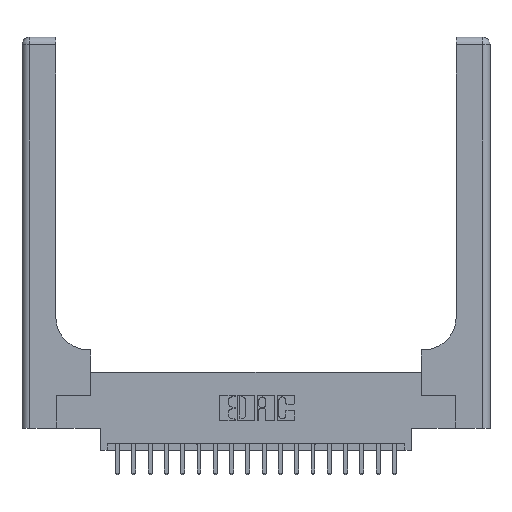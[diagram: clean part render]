
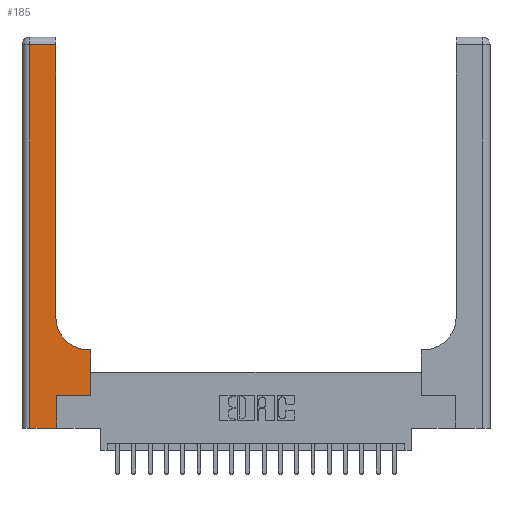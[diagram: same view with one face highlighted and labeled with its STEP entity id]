
A CAD part, top view. The second image highlights one B-rep face of the part: STEP entity #185.
In plain terms, the highlighted planar face has unit normal (0, 0, 1).
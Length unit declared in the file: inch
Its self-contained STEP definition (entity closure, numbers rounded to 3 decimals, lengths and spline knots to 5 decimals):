
#185 = ADVANCED_FACE ( 'NONE', ( #531 ), #16357, .F. ) ;
#223 = EDGE_CURVE ( 'NONE', #10310, #5953, #11863, .T. ) ;
#393 = ORIENTED_EDGE ( 'NONE', *, *, #2539, .T. ) ;
#531 = FACE_OUTER_BOUND ( 'NONE', #19480, .T. ) ;
#795 = ORIENTED_EDGE ( 'NONE', *, *, #9031, .T. ) ;
#1350 = DIRECTION ( 'NONE',  ( 0., 1., 0. ) ) ;
#1409 = ORIENTED_EDGE ( 'NONE', *, *, #223, .T. ) ;
#1670 = CARTESIAN_POINT ( 'NONE',  ( 0., 2.94, 0.37 ) ) ;
#2201 = CARTESIAN_POINT ( 'NONE',  ( 0.528, 0.25, 0.37 ) ) ;
#2447 = ORIENTED_EDGE ( 'NONE', *, *, #11754, .T. ) ;
#2539 = EDGE_CURVE ( 'NONE', #5953, #5606, #13734, .T. ) ;
#2659 = VECTOR ( 'NONE', #10276, 39.37008 ) ;
#2697 = VERTEX_POINT ( 'NONE', #13603 ) ;
#2751 = CARTESIAN_POINT ( 'NONE',  ( 0., 0., 0.37 ) ) ;
#4132 = VERTEX_POINT ( 'NONE', #9927 ) ;
#4357 = DIRECTION ( 'NONE',  ( 1., 0., 0. ) ) ;
#4760 = VECTOR ( 'NONE', #1350, 39.37008 ) ;
#4861 = AXIS2_PLACEMENT_3D ( 'NONE', #6314, #17460, #7933 ) ;
#5235 = VECTOR ( 'NONE', #15338, 39.37008 ) ;
#5336 = CARTESIAN_POINT ( 'NONE',  ( 0.26, 0.85, 0.37 ) ) ;
#5410 = EDGE_CURVE ( 'NONE', #14576, #2697, #15971, .T. ) ;
#5606 = VERTEX_POINT ( 'NONE', #8684 ) ;
#5953 = VERTEX_POINT ( 'NONE', #9588 ) ;
#6120 = VERTEX_POINT ( 'NONE', #5336 ) ;
#6314 = CARTESIAN_POINT ( 'NONE',  ( 0.51, 0.85, 0.37 ) ) ;
#6491 = ORIENTED_EDGE ( 'NONE', *, *, #5410, .T. ) ;
#7428 = VERTEX_POINT ( 'NONE', #19225 ) ;
#7933 = DIRECTION ( 'NONE',  ( 1., 0., 0. ) ) ;
#8323 = LINE ( 'NONE', #2751, #16804 ) ;
#8450 = CARTESIAN_POINT ( 'NONE',  ( 0.26, 2.94, 0.37 ) ) ;
#8684 = CARTESIAN_POINT ( 'NONE',  ( 0.528, 0.25, 0.37 ) ) ;
#8878 = ORIENTED_EDGE ( 'NONE', *, *, #13618, .T. ) ;
#9031 = EDGE_CURVE ( 'NONE', #6120, #14576, #12773, .T. ) ;
#9588 = CARTESIAN_POINT ( 'NONE',  ( 0.265, 0.25, 0.37 ) ) ;
#9653 = AXIS2_PLACEMENT_3D ( 'NONE', #16289, #16247, #16197 ) ;
#9927 = CARTESIAN_POINT ( 'NONE',  ( 0.51, 0.6, 0.37 ) ) ;
#9931 = DIRECTION ( 'NONE',  ( 0., -1., 0. ) ) ;
#9956 = LINE ( 'NONE', #19302, #18325 ) ;
#10052 = CARTESIAN_POINT ( 'NONE',  ( 0.265, 0., 0.37 ) ) ;
#10140 = VERTEX_POINT ( 'NONE', #11273 ) ;
#10276 = DIRECTION ( 'NONE',  ( 0., 1., 0. ) ) ;
#10310 = VERTEX_POINT ( 'NONE', #10052 ) ;
#10400 = LINE ( 'NONE', #18823, #14647 ) ;
#11032 = DIRECTION ( 'NONE',  ( -1., 0., 0. ) ) ;
#11219 = VECTOR ( 'NONE', #14495, 39.37008 ) ;
#11226 = LINE ( 'NONE', #2201, #2659 ) ;
#11273 = CARTESIAN_POINT ( 'NONE',  ( 0.528, 0.6, 0.37 ) ) ;
#11588 = EDGE_CURVE ( 'NONE', #2697, #7428, #9956, .T. ) ;
#11754 = EDGE_CURVE ( 'NONE', #5606, #10140, #11226, .T. ) ;
#11863 = LINE ( 'NONE', #15744, #19614 ) ;
#12126 = CIRCLE ( 'NONE', #4861, 0.25 ) ;
#12198 = ORIENTED_EDGE ( 'NONE', *, *, #11588, .T. ) ;
#12773 = LINE ( 'NONE', #18785, #4760 ) ;
#13057 = EDGE_CURVE ( 'NONE', #10140, #4132, #10400, .T. ) ;
#13603 = CARTESIAN_POINT ( 'NONE',  ( 0.06, 2.94, 0.37 ) ) ;
#13618 = EDGE_CURVE ( 'NONE', #4132, #6120, #12126, .T. ) ;
#13734 = LINE ( 'NONE', #15665, #5235 ) ;
#14495 = DIRECTION ( 'NONE',  ( -1., 0., 0. ) ) ;
#14576 = VERTEX_POINT ( 'NONE', #8450 ) ;
#14647 = VECTOR ( 'NONE', #11032, 39.37008 ) ;
#15229 = EDGE_CURVE ( 'NONE', #7428, #10310, #8323, .T. ) ;
#15338 = DIRECTION ( 'NONE',  ( 1., 0., 0. ) ) ;
#15665 = CARTESIAN_POINT ( 'NONE',  ( 0.265, 0.25, 0.37 ) ) ;
#15671 = DIRECTION ( 'NONE',  ( 0., 1., 0. ) ) ;
#15720 = ORIENTED_EDGE ( 'NONE', *, *, #15229, .T. ) ;
#15744 = CARTESIAN_POINT ( 'NONE',  ( 0.265, 0., 0.37 ) ) ;
#15971 = LINE ( 'NONE', #1670, #11219 ) ;
#16197 = DIRECTION ( 'NONE',  ( -1., 0., 0. ) ) ;
#16247 = DIRECTION ( 'NONE',  ( 0., 0., -1. ) ) ;
#16289 = CARTESIAN_POINT ( 'NONE',  ( 0., 3., 0.37 ) ) ;
#16357 = PLANE ( 'NONE',  #9653 ) ;
#16804 = VECTOR ( 'NONE', #4357, 39.37008 ) ;
#17460 = DIRECTION ( 'NONE',  ( 0., 0., -1. ) ) ;
#18325 = VECTOR ( 'NONE', #9931, 39.37008 ) ;
#18785 = CARTESIAN_POINT ( 'NONE',  ( 0.26, 3., 0.37 ) ) ;
#18823 = CARTESIAN_POINT ( 'NONE',  ( 0.26, 0.6, 0.37 ) ) ;
#19225 = CARTESIAN_POINT ( 'NONE',  ( 0.06, 0., 0.37 ) ) ;
#19302 = CARTESIAN_POINT ( 'NONE',  ( 0.06, 3., 0.37 ) ) ;
#19480 = EDGE_LOOP ( 'NONE', ( #795, #6491, #12198, #15720, #1409, #393, #2447, #19630, #8878 ) ) ;
#19614 = VECTOR ( 'NONE', #15671, 39.37008 ) ;
#19630 = ORIENTED_EDGE ( 'NONE', *, *, #13057, .T. ) ;
